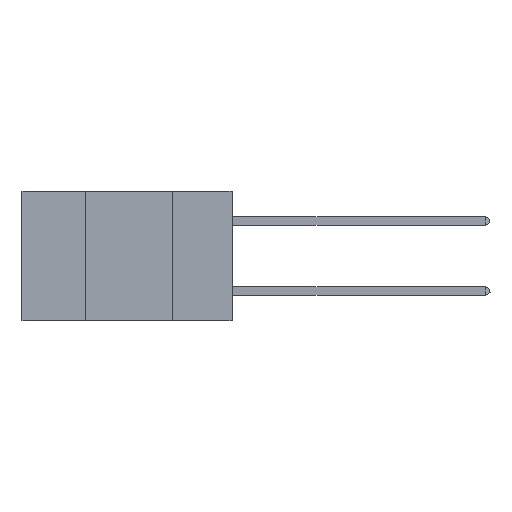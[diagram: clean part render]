
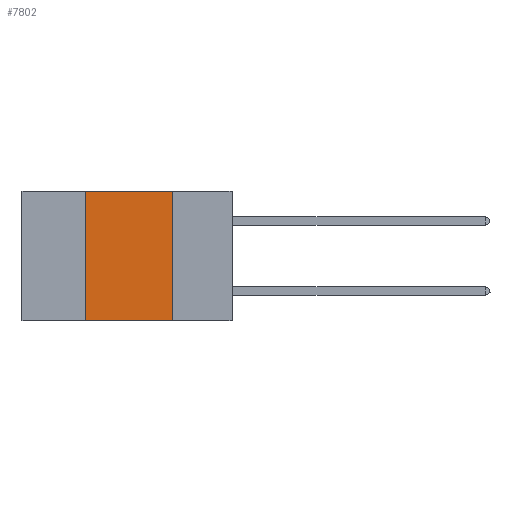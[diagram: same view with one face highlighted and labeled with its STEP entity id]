
A CAD part, left-side view. The second image highlights one B-rep face of the part: STEP entity #7802.
In plain terms, the highlighted planar face has unit normal (-1, 0, 0).
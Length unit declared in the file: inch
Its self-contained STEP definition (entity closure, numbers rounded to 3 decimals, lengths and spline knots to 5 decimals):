
#553 = DIRECTION ( 'NONE',  ( 0., 0., 1. ) ) ;
#646 = DIRECTION ( 'NONE',  ( 1., 0., 0. ) ) ;
#999 = CARTESIAN_POINT ( 'NONE',  ( 0., 0.42, -0.37 ) ) ;
#1983 = VECTOR ( 'NONE', #17084, 39.37008 ) ;
#3036 = EDGE_CURVE ( 'NONE', #15239, #5277, #6547, .T. ) ;
#3108 = AXIS2_PLACEMENT_3D ( 'NONE', #5009, #646, #9518 ) ;
#3243 = VERTEX_POINT ( 'NONE', #999 ) ;
#4311 = EDGE_CURVE ( 'NONE', #3243, #5277, #17212, .T. ) ;
#4343 = EDGE_CURVE ( 'NONE', #3243, #11535, #10460, .T. ) ;
#4434 = CARTESIAN_POINT ( 'NONE',  ( 0., 0.42, 0. ) ) ;
#5009 = CARTESIAN_POINT ( 'NONE',  ( 0., 0.6, 0. ) ) ;
#5248 = CARTESIAN_POINT ( 'NONE',  ( 0., 0.17, 0. ) ) ;
#5277 = VERTEX_POINT ( 'NONE', #15467 ) ;
#5984 = DIRECTION ( 'NONE',  ( 0., 0., -1. ) ) ;
#6195 = VECTOR ( 'NONE', #10815, 39.37008 ) ;
#6547 = LINE ( 'NONE', #13410, #15168 ) ;
#7802 = ADVANCED_FACE ( 'NONE', ( #13058 ), #8219, .F. ) ;
#8219 = PLANE ( 'NONE',  #3108 ) ;
#9518 = DIRECTION ( 'NONE',  ( 0., 0., -1. ) ) ;
#10460 = LINE ( 'NONE', #18519, #13244 ) ;
#10674 = EDGE_CURVE ( 'NONE', #11535, #15239, #11529, .T. ) ;
#10815 = DIRECTION ( 'NONE',  ( 0., -1., 0. ) ) ;
#11529 = LINE ( 'NONE', #19183, #6195 ) ;
#11535 = VERTEX_POINT ( 'NONE', #4434 ) ;
#12016 = ORIENTED_EDGE ( 'NONE', *, *, #3036, .F. ) ;
#12626 = CARTESIAN_POINT ( 'NONE',  ( 0., 0.6, -0.37 ) ) ;
#13058 = FACE_OUTER_BOUND ( 'NONE', #19118, .T. ) ;
#13244 = VECTOR ( 'NONE', #553, 39.37008 ) ;
#13410 = CARTESIAN_POINT ( 'NONE',  ( 0., 0.17, 0. ) ) ;
#14217 = ORIENTED_EDGE ( 'NONE', *, *, #4343, .F. ) ;
#15168 = VECTOR ( 'NONE', #5984, 39.37008 ) ;
#15239 = VERTEX_POINT ( 'NONE', #5248 ) ;
#15467 = CARTESIAN_POINT ( 'NONE',  ( 0., 0.17, -0.37 ) ) ;
#16645 = ORIENTED_EDGE ( 'NONE', *, *, #10674, .F. ) ;
#17084 = DIRECTION ( 'NONE',  ( 0., -1., 0. ) ) ;
#17212 = LINE ( 'NONE', #12626, #1983 ) ;
#18519 = CARTESIAN_POINT ( 'NONE',  ( 0., 0.42, 0. ) ) ;
#19118 = EDGE_LOOP ( 'NONE', ( #12016, #16645, #14217, #19398 ) ) ;
#19183 = CARTESIAN_POINT ( 'NONE',  ( 0., 0.6, 0. ) ) ;
#19398 = ORIENTED_EDGE ( 'NONE', *, *, #4311, .T. ) ;
